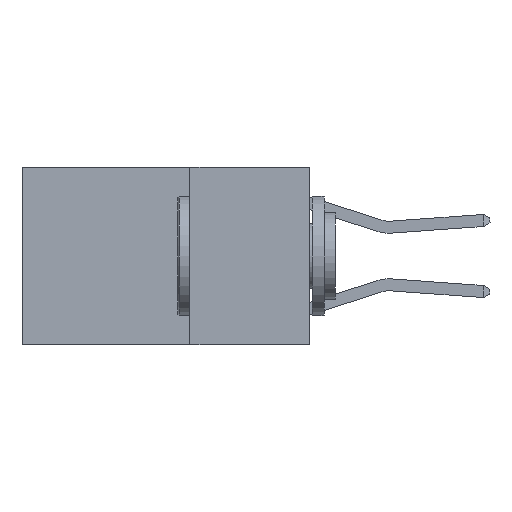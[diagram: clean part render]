
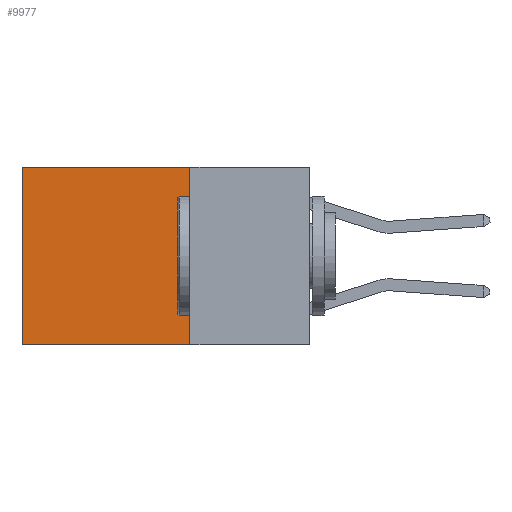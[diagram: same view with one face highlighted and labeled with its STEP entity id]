
A CAD part, left-side view. The second image highlights one B-rep face of the part: STEP entity #9977.
In plain terms, the highlighted planar face has unit normal (-1, 0, 0).
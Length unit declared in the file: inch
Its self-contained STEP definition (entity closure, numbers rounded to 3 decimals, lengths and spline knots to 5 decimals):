
#94 = VECTOR ( 'NONE', #16598, 39.37008 ) ;
#491 = LINE ( 'NONE', #8667, #1627 ) ;
#826 = CARTESIAN_POINT ( 'NONE',  ( 0.2625, 0.6, 0. ) ) ;
#1627 = VECTOR ( 'NONE', #11215, 39.37008 ) ;
#1790 = VERTEX_POINT ( 'NONE', #14443 ) ;
#2282 = EDGE_LOOP ( 'NONE', ( #14970, #10674, #5525, #10793 ) ) ;
#2386 = EDGE_CURVE ( 'NONE', #14741, #6997, #11511, .T. ) ;
#5525 = ORIENTED_EDGE ( 'NONE', *, *, #2386, .F. ) ;
#6413 = LINE ( 'NONE', #8303, #14561 ) ;
#6997 = VERTEX_POINT ( 'NONE', #9919 ) ;
#7092 = EDGE_CURVE ( 'NONE', #14741, #9843, #491, .T. ) ;
#8070 = EDGE_CURVE ( 'NONE', #9843, #1790, #6413, .T. ) ;
#8292 = DIRECTION ( 'NONE',  ( 1., 0., 0. ) ) ;
#8303 = CARTESIAN_POINT ( 'NONE',  ( 0.2625, 0.6, 0. ) ) ;
#8667 = CARTESIAN_POINT ( 'NONE',  ( 0.2625, 0.25, 0. ) ) ;
#9084 = VECTOR ( 'NONE', #13900, 39.37008 ) ;
#9558 = PLANE ( 'NONE',  #14245 ) ;
#9843 = VERTEX_POINT ( 'NONE', #826 ) ;
#9919 = CARTESIAN_POINT ( 'NONE',  ( 0.2625, 0.25, -0.37 ) ) ;
#9977 = ADVANCED_FACE ( 'NONE', ( #12597 ), #9558, .F. ) ;
#10397 = LINE ( 'NONE', #15196, #94 ) ;
#10674 = ORIENTED_EDGE ( 'NONE', *, *, #15819, .F. ) ;
#10793 = ORIENTED_EDGE ( 'NONE', *, *, #7092, .T. ) ;
#10813 = DIRECTION ( 'NONE',  ( 0., 0., -1. ) ) ;
#10909 = DIRECTION ( 'NONE',  ( 0., 0., -1. ) ) ;
#11215 = DIRECTION ( 'NONE',  ( 0., 1., 0. ) ) ;
#11511 = LINE ( 'NONE', #15401, #9084 ) ;
#12597 = FACE_OUTER_BOUND ( 'NONE', #2282, .T. ) ;
#13900 = DIRECTION ( 'NONE',  ( 0., 0., -1. ) ) ;
#14245 = AXIS2_PLACEMENT_3D ( 'NONE', #16089, #8292, #10909 ) ;
#14443 = CARTESIAN_POINT ( 'NONE',  ( 0.2625, 0.6, -0.37 ) ) ;
#14561 = VECTOR ( 'NONE', #10813, 39.37008 ) ;
#14741 = VERTEX_POINT ( 'NONE', #16751 ) ;
#14970 = ORIENTED_EDGE ( 'NONE', *, *, #8070, .T. ) ;
#15196 = CARTESIAN_POINT ( 'NONE',  ( 0.2625, 0.25, -0.37 ) ) ;
#15401 = CARTESIAN_POINT ( 'NONE',  ( 0.2625, 0.25, 0. ) ) ;
#15819 = EDGE_CURVE ( 'NONE', #6997, #1790, #10397, .T. ) ;
#16089 = CARTESIAN_POINT ( 'NONE',  ( 0.2625, 0.25, 0. ) ) ;
#16598 = DIRECTION ( 'NONE',  ( 0., 1., 0. ) ) ;
#16751 = CARTESIAN_POINT ( 'NONE',  ( 0.2625, 0.25, 0. ) ) ;
